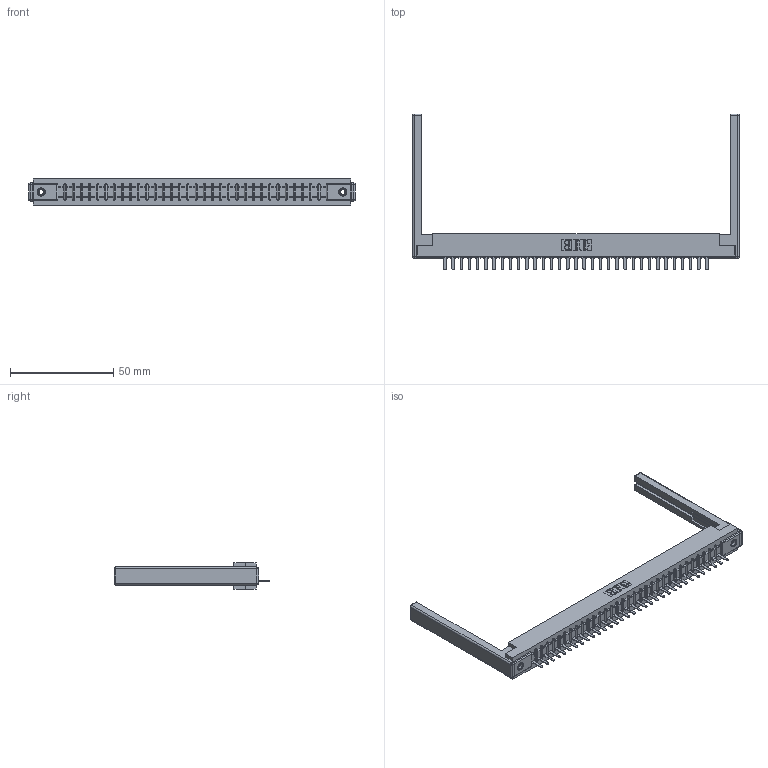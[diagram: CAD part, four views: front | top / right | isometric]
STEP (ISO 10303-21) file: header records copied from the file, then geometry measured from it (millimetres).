
FILE_DESCRIPTION (( 'STEP AP203' ), '1' );
FILE_NAME ('307-033-421-168.STEP', '2020-09-28T19:22:42', ( '' ), ( '' ), 'SwSTEP 2.0', 'SolidWorks 2020', '' );
FILE_SCHEMA (( 'CONFIG_CONTROL_DESIGN' ));
Length unit declared in the file: inch
Products named in the file (5): 307-290-002_521; 307 Part_.156 Dia Mounting Holes; 307-220-068; 345-250-001_345-250-001-102; 307-033-421-168
Assembly tree (38 placements, depth 2):
  307-033-421-168
    307 Part_.156 Dia Mounting Holes
    307-290-002_521  x33
    307-220-068  x2
    345-250-001_345-250-001-102  x2
Bounding box: 158.19 x 75.39 x 12.7 mm (x, y, z)
Volume: 21240.9 mm3; surface area: 24972.8 mm2
Topology: 38 solids, 38 shells, 2748 faces, 8369 edges, 5466 vertices
Faces by surface type: plane 1643, cylinder 1013, sphere 76, cone 12, torus 4
Entity records: 32877 total; most frequent: CARTESIAN_POINT 5509, ORIENTED_EDGE 5488, DIRECTION 5374, EDGE_CURVE 2744, VECTOR 2096, LINE 2096, VERTEX_POINT 1774, AXIS2_PLACEMENT_3D 1639
